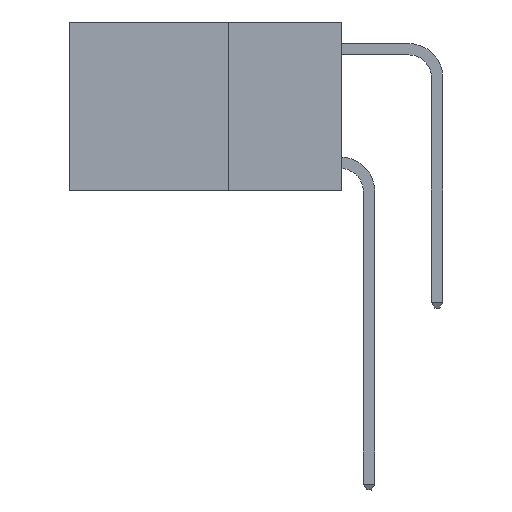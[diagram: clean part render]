
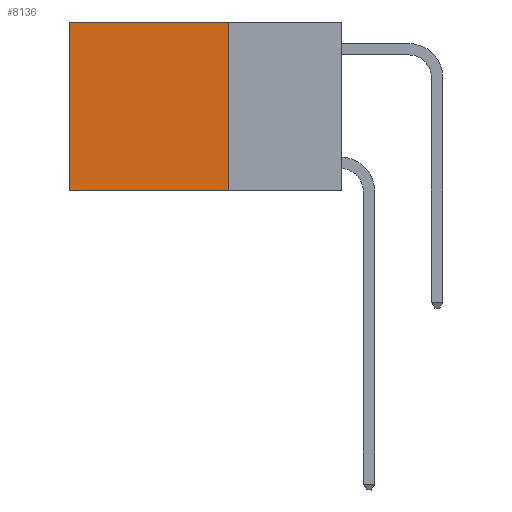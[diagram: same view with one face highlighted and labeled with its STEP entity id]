
A CAD part, left-side view. The second image highlights one B-rep face of the part: STEP entity #8136.
In plain terms, the highlighted planar face has unit normal (-1, 0, 0).
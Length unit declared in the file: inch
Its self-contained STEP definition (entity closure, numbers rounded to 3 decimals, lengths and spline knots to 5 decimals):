
#301 = EDGE_CURVE ( 'NONE', #12653, #8781, #1299, .T. ) ;
#805 = CARTESIAN_POINT ( 'NONE',  ( 0.2625, 0.25, 0. ) ) ;
#1226 = CARTESIAN_POINT ( 'NONE',  ( 0.2625, 0.25, 0. ) ) ;
#1299 = LINE ( 'NONE', #4131, #12628 ) ;
#1785 = LINE ( 'NONE', #4360, #10442 ) ;
#1794 = EDGE_CURVE ( 'NONE', #12329, #3078, #6173, .T. ) ;
#1931 = EDGE_LOOP ( 'NONE', ( #8738, #10836, #7304, #13191 ) ) ;
#2981 = EDGE_CURVE ( 'NONE', #8781, #3078, #1785, .T. ) ;
#3078 = VERTEX_POINT ( 'NONE', #14271 ) ;
#3185 = DIRECTION ( 'NONE',  ( 0., 0., -1. ) ) ;
#3768 = PLANE ( 'NONE',  #5980 ) ;
#4131 = CARTESIAN_POINT ( 'NONE',  ( 0.2625, 0.25, 0. ) ) ;
#4360 = CARTESIAN_POINT ( 'NONE',  ( 0.2625, 0.6, 0. ) ) ;
#4897 = DIRECTION ( 'NONE',  ( 1., 0., 0. ) ) ;
#5068 = CARTESIAN_POINT ( 'NONE',  ( 0.2625, 0.25, -0.37 ) ) ;
#5352 = DIRECTION ( 'NONE',  ( 0., 1., 0. ) ) ;
#5980 = AXIS2_PLACEMENT_3D ( 'NONE', #1226, #4897, #12612 ) ;
#6173 = LINE ( 'NONE', #11963, #9140 ) ;
#6506 = CARTESIAN_POINT ( 'NONE',  ( 0.2625, 0.25, 0. ) ) ;
#6616 = VECTOR ( 'NONE', #7818, 39.37008 ) ;
#6814 = CARTESIAN_POINT ( 'NONE',  ( 0.2625, 0.6, 0. ) ) ;
#7304 = ORIENTED_EDGE ( 'NONE', *, *, #13562, .F. ) ;
#7818 = DIRECTION ( 'NONE',  ( 0., 0., -1. ) ) ;
#8136 = ADVANCED_FACE ( 'NONE', ( #13773 ), #3768, .F. ) ;
#8738 = ORIENTED_EDGE ( 'NONE', *, *, #2981, .T. ) ;
#8781 = VERTEX_POINT ( 'NONE', #6814 ) ;
#9140 = VECTOR ( 'NONE', #5352, 39.37008 ) ;
#9570 = LINE ( 'NONE', #805, #6616 ) ;
#10442 = VECTOR ( 'NONE', #3185, 39.37008 ) ;
#10836 = ORIENTED_EDGE ( 'NONE', *, *, #1794, .F. ) ;
#11781 = DIRECTION ( 'NONE',  ( 0., 1., 0. ) ) ;
#11963 = CARTESIAN_POINT ( 'NONE',  ( 0.2625, 0.25, -0.37 ) ) ;
#12329 = VERTEX_POINT ( 'NONE', #5068 ) ;
#12612 = DIRECTION ( 'NONE',  ( 0., 0., -1. ) ) ;
#12628 = VECTOR ( 'NONE', #11781, 39.37008 ) ;
#12653 = VERTEX_POINT ( 'NONE', #6506 ) ;
#13191 = ORIENTED_EDGE ( 'NONE', *, *, #301, .T. ) ;
#13562 = EDGE_CURVE ( 'NONE', #12653, #12329, #9570, .T. ) ;
#13773 = FACE_OUTER_BOUND ( 'NONE', #1931, .T. ) ;
#14271 = CARTESIAN_POINT ( 'NONE',  ( 0.2625, 0.6, -0.37 ) ) ;
